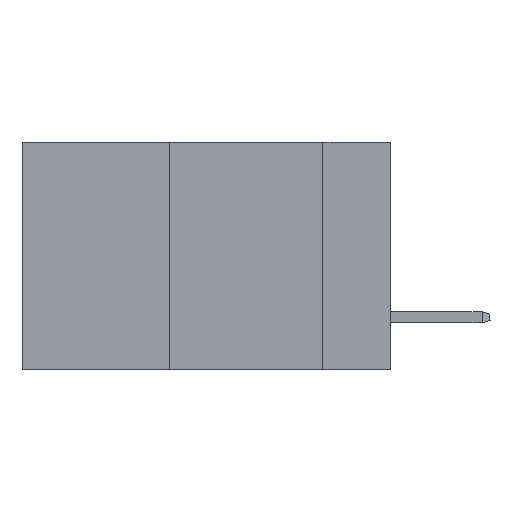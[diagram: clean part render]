
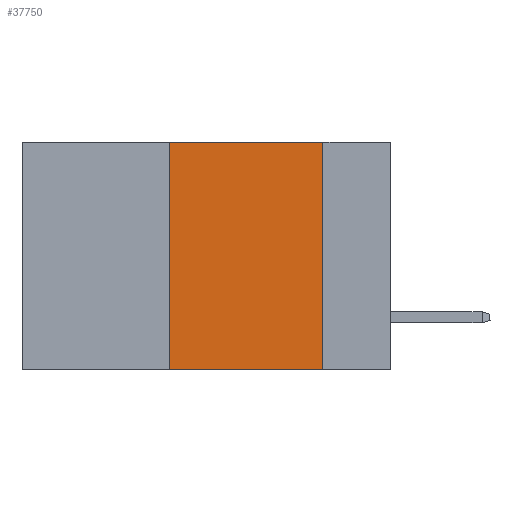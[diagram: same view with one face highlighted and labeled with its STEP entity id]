
A CAD part, left-side view. The second image highlights one B-rep face of the part: STEP entity #37750.
In plain terms, the highlighted planar face has unit normal (-1, 0, 0).
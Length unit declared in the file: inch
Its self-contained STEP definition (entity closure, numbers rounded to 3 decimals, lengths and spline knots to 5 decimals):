
#1534 = LINE ( 'NONE', #16828, #32360 ) ;
#1684 = ORIENTED_EDGE ( 'NONE', *, *, #39475, .T. ) ;
#1759 = EDGE_LOOP ( 'NONE', ( #27142, #18630, #34630, #1684 ) ) ;
#2135 = CARTESIAN_POINT ( 'NONE',  ( 0., 0.36, 0. ) ) ;
#2752 = CARTESIAN_POINT ( 'NONE',  ( 0., 0.36, -0.37 ) ) ;
#2900 = DIRECTION ( 'NONE',  ( 0., 0., -1. ) ) ;
#2922 = CARTESIAN_POINT ( 'NONE',  ( 0., 0.11, -0.37 ) ) ;
#7590 = DIRECTION ( 'NONE',  ( 0., 0., -1. ) ) ;
#8084 = LINE ( 'NONE', #14580, #27958 ) ;
#8195 = VERTEX_POINT ( 'NONE', #2752 ) ;
#9637 = PLANE ( 'NONE',  #13371 ) ;
#9753 = VERTEX_POINT ( 'NONE', #2135 ) ;
#10706 = DIRECTION ( 'NONE',  ( 0., -1., 0. ) ) ;
#12262 = LINE ( 'NONE', #24736, #28779 ) ;
#12895 = CARTESIAN_POINT ( 'NONE',  ( 0., 0.6, 0. ) ) ;
#13371 = AXIS2_PLACEMENT_3D ( 'NONE', #12895, #40195, #2900 ) ;
#14580 = CARTESIAN_POINT ( 'NONE',  ( 0., 0.36, 0. ) ) ;
#16281 = CARTESIAN_POINT ( 'NONE',  ( 0., 0.11, 0. ) ) ;
#16828 = CARTESIAN_POINT ( 'NONE',  ( 0., 0.6, -0.37 ) ) ;
#18630 = ORIENTED_EDGE ( 'NONE', *, *, #30270, .F. ) ;
#18909 = VERTEX_POINT ( 'NONE', #16281 ) ;
#20864 = VECTOR ( 'NONE', #35704, 39.37008 ) ;
#24736 = CARTESIAN_POINT ( 'NONE',  ( 0., 0.11, 0. ) ) ;
#26564 = LINE ( 'NONE', #33054, #20864 ) ;
#27142 = ORIENTED_EDGE ( 'NONE', *, *, #32058, .F. ) ;
#27958 = VECTOR ( 'NONE', #35239, 39.37008 ) ;
#28779 = VECTOR ( 'NONE', #7590, 39.37008 ) ;
#29416 = EDGE_CURVE ( 'NONE', #8195, #9753, #8084, .T. ) ;
#30270 = EDGE_CURVE ( 'NONE', #9753, #18909, #26564, .T. ) ;
#30833 = FACE_OUTER_BOUND ( 'NONE', #1759, .T. ) ;
#31112 = VERTEX_POINT ( 'NONE', #2922 ) ;
#32058 = EDGE_CURVE ( 'NONE', #18909, #31112, #12262, .T. ) ;
#32360 = VECTOR ( 'NONE', #10706, 39.37008 ) ;
#33054 = CARTESIAN_POINT ( 'NONE',  ( 0., 0.6, 0. ) ) ;
#34630 = ORIENTED_EDGE ( 'NONE', *, *, #29416, .F. ) ;
#35239 = DIRECTION ( 'NONE',  ( 0., 0., 1. ) ) ;
#35704 = DIRECTION ( 'NONE',  ( 0., -1., 0. ) ) ;
#37750 = ADVANCED_FACE ( 'NONE', ( #30833 ), #9637, .F. ) ;
#39475 = EDGE_CURVE ( 'NONE', #8195, #31112, #1534, .T. ) ;
#40195 = DIRECTION ( 'NONE',  ( 1., 0., 0. ) ) ;
